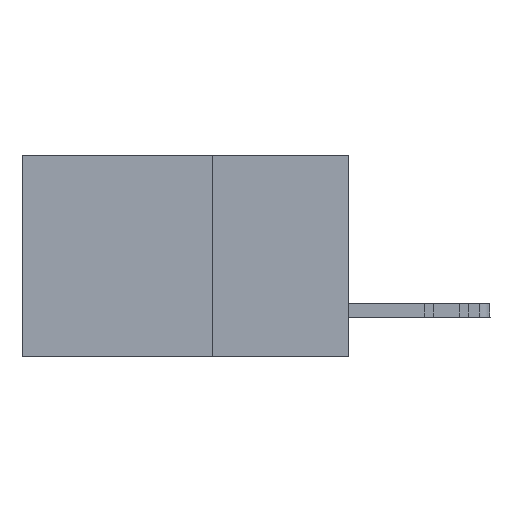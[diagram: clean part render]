
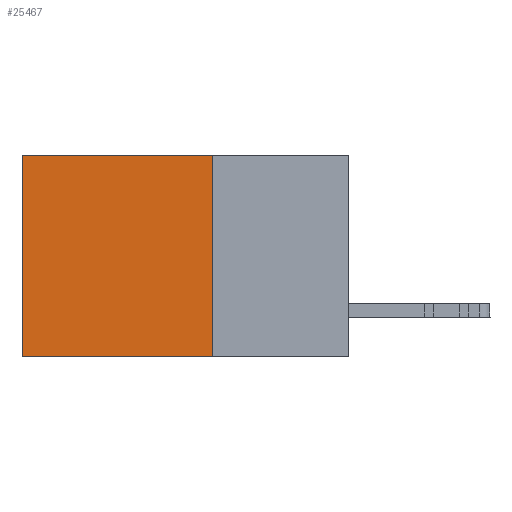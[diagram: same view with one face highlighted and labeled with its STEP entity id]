
A CAD part, left-side view. The second image highlights one B-rep face of the part: STEP entity #25467.
In plain terms, the highlighted planar face has unit normal (-1, 0, 0).
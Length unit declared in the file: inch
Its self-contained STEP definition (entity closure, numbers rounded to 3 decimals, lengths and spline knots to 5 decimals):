
#5275 = EDGE_CURVE ( 'NONE', #7460, #18709, #23025, .T. ) ;
#5342 = CARTESIAN_POINT ( 'NONE',  ( 0.298, 0.25, 0. ) ) ;
#6568 = DIRECTION ( 'NONE',  ( 0., 0., -1. ) ) ;
#7366 = VERTEX_POINT ( 'NONE', #12382 ) ;
#7460 = VERTEX_POINT ( 'NONE', #17884 ) ;
#8131 = CARTESIAN_POINT ( 'NONE',  ( 0.298, 0.6, -0.37 ) ) ;
#9249 = CARTESIAN_POINT ( 'NONE',  ( 0.298, 0.25, 0. ) ) ;
#9350 = ORIENTED_EDGE ( 'NONE', *, *, #21147, .T. ) ;
#11067 = VECTOR ( 'NONE', #27380, 39.37008 ) ;
#11794 = EDGE_CURVE ( 'NONE', #7366, #18793, #12969, .T. ) ;
#12132 = VECTOR ( 'NONE', #6568, 39.37008 ) ;
#12160 = DIRECTION ( 'NONE',  ( 0., 0., -1. ) ) ;
#12382 = CARTESIAN_POINT ( 'NONE',  ( 0.298, 0.25, 0. ) ) ;
#12969 = LINE ( 'NONE', #5342, #23845 ) ;
#13255 = ORIENTED_EDGE ( 'NONE', *, *, #11794, .T. ) ;
#13965 = VECTOR ( 'NONE', #12160, 39.37008 ) ;
#14467 = ORIENTED_EDGE ( 'NONE', *, *, #17109, .F. ) ;
#16667 = AXIS2_PLACEMENT_3D ( 'NONE', #9249, #28971, #16707 ) ;
#16705 = LINE ( 'NONE', #29120, #12132 ) ;
#16707 = DIRECTION ( 'NONE',  ( 0., 0., -1. ) ) ;
#17109 = EDGE_CURVE ( 'NONE', #7366, #7460, #16705, .T. ) ;
#17884 = CARTESIAN_POINT ( 'NONE',  ( 0.298, 0.25, -0.37 ) ) ;
#18709 = VERTEX_POINT ( 'NONE', #8131 ) ;
#18793 = VERTEX_POINT ( 'NONE', #26837 ) ;
#20365 = CARTESIAN_POINT ( 'NONE',  ( 0.298, 0.25, -0.37 ) ) ;
#20661 = LINE ( 'NONE', #21111, #13965 ) ;
#21111 = CARTESIAN_POINT ( 'NONE',  ( 0.298, 0.6, 0. ) ) ;
#21147 = EDGE_CURVE ( 'NONE', #18793, #18709, #20661, .T. ) ;
#21216 = DIRECTION ( 'NONE',  ( 0., 1., 0. ) ) ;
#22780 = EDGE_LOOP ( 'NONE', ( #9350, #29094, #14467, #13255 ) ) ;
#22868 = FACE_OUTER_BOUND ( 'NONE', #22780, .T. ) ;
#23025 = LINE ( 'NONE', #20365, #11067 ) ;
#23845 = VECTOR ( 'NONE', #21216, 39.37008 ) ;
#25467 = ADVANCED_FACE ( 'NONE', ( #22868 ), #27679, .F. ) ;
#26837 = CARTESIAN_POINT ( 'NONE',  ( 0.298, 0.6, 0. ) ) ;
#27380 = DIRECTION ( 'NONE',  ( 0., 1., 0. ) ) ;
#27679 = PLANE ( 'NONE',  #16667 ) ;
#28971 = DIRECTION ( 'NONE',  ( 1., 0., 0. ) ) ;
#29094 = ORIENTED_EDGE ( 'NONE', *, *, #5275, .F. ) ;
#29120 = CARTESIAN_POINT ( 'NONE',  ( 0.298, 0.25, 0. ) ) ;
